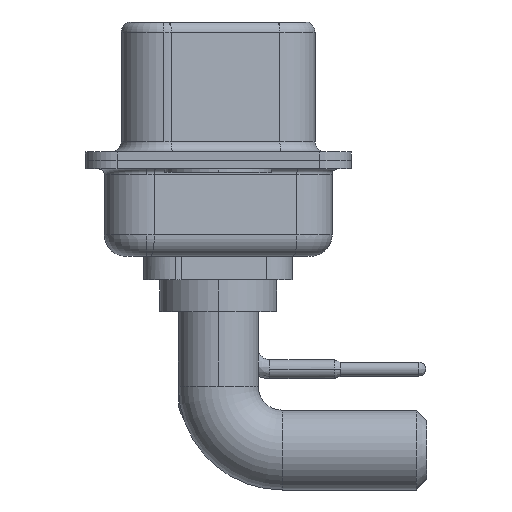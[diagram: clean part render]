
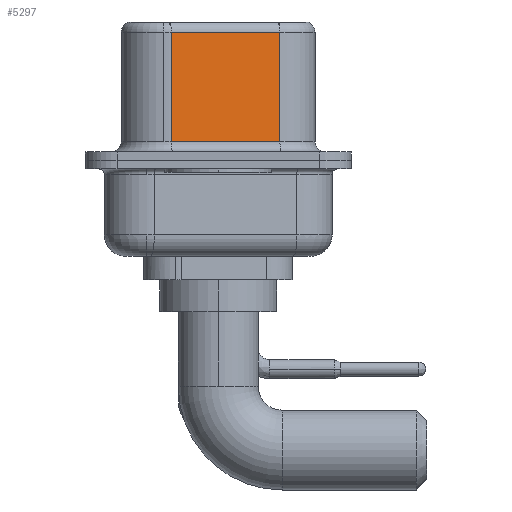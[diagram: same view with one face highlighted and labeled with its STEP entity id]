
A CAD part, left-side view. The second image highlights one B-rep face of the part: STEP entity #5297.
In plain terms, the highlighted planar face has unit normal (-0.985, -0.174, 0).
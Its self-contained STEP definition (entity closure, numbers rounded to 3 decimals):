
#422 = CARTESIAN_POINT ( 'NONE',  ( 4.58, -2.897, 6.52 ) ) ;
#1806 = VERTEX_POINT ( 'NONE', #15560 ) ;
#2562 = VERTEX_POINT ( 'NONE', #14243 ) ;
#2700 = ORIENTED_EDGE ( 'NONE', *, *, #18365, .T. ) ;
#3194 = LINE ( 'NONE', #22670, #11868 ) ;
#4451 = LINE ( 'NONE', #11659, #15533 ) ;
#5066 = DIRECTION ( 'NONE',  ( -0.174, 0.985, 0. ) ) ;
#5297 = ADVANCED_FACE ( 'NONE', ( #6979 ), #21594, .F. ) ;
#6144 = CARTESIAN_POINT ( 'NONE',  ( 4.58, -2.897, 6.02 ) ) ;
#6349 = DIRECTION ( 'NONE',  ( 0., 0., -1. ) ) ;
#6474 = LINE ( 'NONE', #8045, #12212 ) ;
#6686 = DIRECTION ( 'NONE',  ( 0.174, -0.985, 0. ) ) ;
#6979 = FACE_OUTER_BOUND ( 'NONE', #16325, .T. ) ;
#8045 = CARTESIAN_POINT ( 'NONE',  ( 3.68, 2.203, 6.52 ) ) ;
#8299 = DIRECTION ( 'NONE',  ( -0.174, 0.985, 0. ) ) ;
#8949 = VECTOR ( 'NONE', #13303, 1000. ) ;
#11659 = CARTESIAN_POINT ( 'NONE',  ( 4.58, -2.897, 6.02 ) ) ;
#11868 = VECTOR ( 'NONE', #6686, 1000. ) ;
#12212 = VECTOR ( 'NONE', #6349, 1000. ) ;
#13303 = DIRECTION ( 'NONE',  ( 0., 0., -1. ) ) ;
#14243 = CARTESIAN_POINT ( 'NONE',  ( 3.68, 2.203, 0.9 ) ) ;
#15232 = AXIS2_PLACEMENT_3D ( 'NONE', #23065, #21490, #5066 ) ;
#15263 = EDGE_CURVE ( 'NONE', #21896, #1806, #4451, .T. ) ;
#15533 = VECTOR ( 'NONE', #8299, 1000. ) ;
#15560 = CARTESIAN_POINT ( 'NONE',  ( 3.68, 2.203, 6.02 ) ) ;
#16325 = EDGE_LOOP ( 'NONE', ( #20198, #17795, #2700, #17089 ) ) ;
#17089 = ORIENTED_EDGE ( 'NONE', *, *, #20716, .T. ) ;
#17795 = ORIENTED_EDGE ( 'NONE', *, *, #15263, .T. ) ;
#18365 = EDGE_CURVE ( 'NONE', #1806, #2562, #6474, .T. ) ;
#18857 = LINE ( 'NONE', #422, #8949 ) ;
#19807 = CARTESIAN_POINT ( 'NONE',  ( 4.58, -2.897, 0.9 ) ) ;
#20198 = ORIENTED_EDGE ( 'NONE', *, *, #21066, .F. ) ;
#20716 = EDGE_CURVE ( 'NONE', #2562, #21290, #3194, .T. ) ;
#21066 = EDGE_CURVE ( 'NONE', #21896, #21290, #18857, .T. ) ;
#21290 = VERTEX_POINT ( 'NONE', #19807 ) ;
#21490 = DIRECTION ( 'NONE',  ( 0.985, 0.174, 0. ) ) ;
#21594 = PLANE ( 'NONE',  #15232 ) ;
#21896 = VERTEX_POINT ( 'NONE', #6144 ) ;
#22670 = CARTESIAN_POINT ( 'NONE',  ( 4.58, -2.897, 0.9 ) ) ;
#23065 = CARTESIAN_POINT ( 'NONE',  ( 4.58, -2.897, 6.52 ) ) ;
